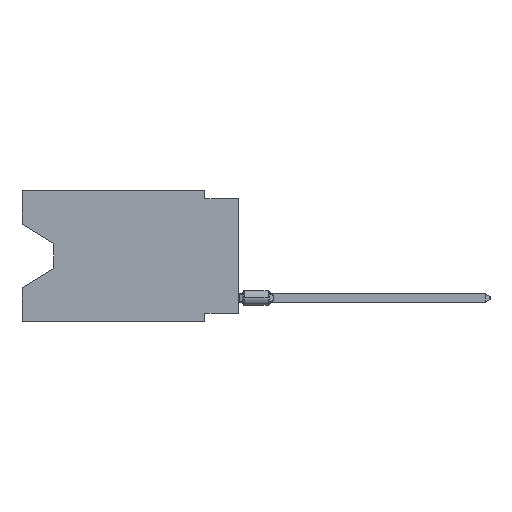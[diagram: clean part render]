
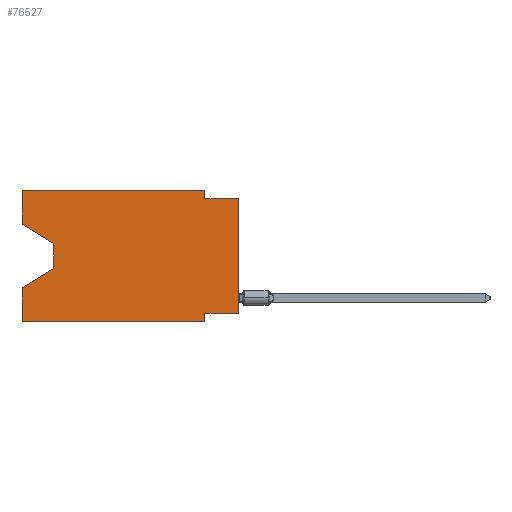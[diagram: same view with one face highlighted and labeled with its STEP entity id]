
A CAD part, left-side view. The second image highlights one B-rep face of the part: STEP entity #76527.
In plain terms, the highlighted planar face has unit normal (-1, 0, 0).
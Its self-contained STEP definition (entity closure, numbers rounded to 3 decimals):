
#252 = DIRECTION ( 'NONE',  ( 0., -1., 0. ) ) ;
#320 = DIRECTION ( 'NONE',  ( 0., 0., 1. ) ) ;
#883 = CARTESIAN_POINT ( 'NONE',  ( 0., 16.383, 0. ) ) ;
#2734 = VERTEX_POINT ( 'NONE', #69233 ) ;
#3400 = VERTEX_POINT ( 'NONE', #31147 ) ;
#4760 = CARTESIAN_POINT ( 'NONE',  ( 0., 13.97, -4.013 ) ) ;
#5034 = EDGE_CURVE ( 'NONE', #14132, #26590, #78920, .T. ) ;
#6052 = VECTOR ( 'NONE', #58578, 1000. ) ;
#8545 = EDGE_CURVE ( 'NONE', #2734, #3400, #18731, .T. ) ;
#8686 = EDGE_CURVE ( 'NONE', #66600, #31402, #77104, .T. ) ;
#9120 = FACE_OUTER_BOUND ( 'NONE', #32120, .T. ) ;
#9383 = CARTESIAN_POINT ( 'NONE',  ( 0., 16.383, -2.546 ) ) ;
#10279 = VERTEX_POINT ( 'NONE', #65061 ) ;
#11638 = ORIENTED_EDGE ( 'NONE', *, *, #46056, .F. ) ;
#11799 = CARTESIAN_POINT ( 'NONE',  ( 0., 16.383, -9.906 ) ) ;
#11933 = LINE ( 'NONE', #24694, #43469 ) ;
#11943 = CARTESIAN_POINT ( 'NONE',  ( 0., 2.54, -9.906 ) ) ;
#12550 = AXIS2_PLACEMENT_3D ( 'NONE', #46155, #47347, #40383 ) ;
#13216 = LINE ( 'NONE', #883, #72345 ) ;
#13653 = VERTEX_POINT ( 'NONE', #71259 ) ;
#14021 = DIRECTION ( 'NONE',  ( 0., 0., 1. ) ) ;
#14132 = VERTEX_POINT ( 'NONE', #9383 ) ;
#14523 = CARTESIAN_POINT ( 'NONE',  ( 0., 16.383, 0. ) ) ;
#14985 = CARTESIAN_POINT ( 'NONE',  ( 0., 16.383, -9.906 ) ) ;
#15037 = ORIENTED_EDGE ( 'NONE', *, *, #69292, .T. ) ;
#18731 = LINE ( 'NONE', #63143, #41501 ) ;
#20575 = EDGE_CURVE ( 'NONE', #66600, #42557, #48158, .T. ) ;
#20995 = ORIENTED_EDGE ( 'NONE', *, *, #8545, .F. ) ;
#21730 = ORIENTED_EDGE ( 'NONE', *, *, #49374, .T. ) ;
#22168 = ORIENTED_EDGE ( 'NONE', *, *, #8686, .T. ) ;
#23482 = DIRECTION ( 'NONE',  ( 0., 0., 1. ) ) ;
#23581 = EDGE_CURVE ( 'NONE', #80681, #2734, #27623, .T. ) ;
#23883 = CARTESIAN_POINT ( 'NONE',  ( 0., 2.54, 0. ) ) ;
#24074 = LINE ( 'NONE', #4760, #71920 ) ;
#24694 = CARTESIAN_POINT ( 'NONE',  ( 0., 13.97, -5.893 ) ) ;
#25001 = VECTOR ( 'NONE', #39782, 1000. ) ;
#25594 = VERTEX_POINT ( 'NONE', #27034 ) ;
#26219 = CARTESIAN_POINT ( 'NONE',  ( 0., 0., -9.271 ) ) ;
#26590 = VERTEX_POINT ( 'NONE', #40401 ) ;
#27034 = CARTESIAN_POINT ( 'NONE',  ( 0., 13.97, -5.893 ) ) ;
#27076 = VECTOR ( 'NONE', #62102, 1000. ) ;
#27623 = LINE ( 'NONE', #63812, #40417 ) ;
#28170 = ORIENTED_EDGE ( 'NONE', *, *, #51060, .T. ) ;
#28357 = CARTESIAN_POINT ( 'NONE',  ( 0., 16.383, -2.546 ) ) ;
#30069 = VECTOR ( 'NONE', #320, 1000. ) ;
#31147 = CARTESIAN_POINT ( 'NONE',  ( 0., 0., -0.635 ) ) ;
#31402 = VERTEX_POINT ( 'NONE', #54485 ) ;
#32120 = EDGE_LOOP ( 'NONE', ( #36645, #21730, #15037, #40315, #22168, #11638, #81163, #28170, #20995, #37287, #57094, #35617 ) ) ;
#35617 = ORIENTED_EDGE ( 'NONE', *, *, #55524, .F. ) ;
#36645 = ORIENTED_EDGE ( 'NONE', *, *, #5034, .T. ) ;
#37287 = ORIENTED_EDGE ( 'NONE', *, *, #23581, .F. ) ;
#37332 = LINE ( 'NONE', #68564, #30069 ) ;
#39782 = DIRECTION ( 'NONE',  ( 0., 1., 0. ) ) ;
#40315 = ORIENTED_EDGE ( 'NONE', *, *, #20575, .F. ) ;
#40383 = DIRECTION ( 'NONE',  ( 0., 0., -1. ) ) ;
#40401 = CARTESIAN_POINT ( 'NONE',  ( 0., 13.97, -4.013 ) ) ;
#40417 = VECTOR ( 'NONE', #58065, 1000. ) ;
#41501 = VECTOR ( 'NONE', #252, 1000. ) ;
#42437 = DIRECTION ( 'NONE',  ( 0., -1., 0. ) ) ;
#42557 = VERTEX_POINT ( 'NONE', #77464 ) ;
#43469 = VECTOR ( 'NONE', #74847, 1000. ) ;
#45945 = LINE ( 'NONE', #26219, #25001 ) ;
#46056 = EDGE_CURVE ( 'NONE', #64828, #31402, #68265, .T. ) ;
#46155 = CARTESIAN_POINT ( 'NONE',  ( 0., 16.383, 0. ) ) ;
#47347 = DIRECTION ( 'NONE',  ( 1., 0., 0. ) ) ;
#48158 = LINE ( 'NONE', #72816, #77491 ) ;
#49270 = VECTOR ( 'NONE', #42437, 1000. ) ;
#49374 = EDGE_CURVE ( 'NONE', #26590, #25594, #24074, .T. ) ;
#51060 = EDGE_CURVE ( 'NONE', #13653, #3400, #37332, .T. ) ;
#52389 = EDGE_CURVE ( 'NONE', #13653, #64828, #45945, .T. ) ;
#54485 = CARTESIAN_POINT ( 'NONE',  ( 0., 2.54, -9.906 ) ) ;
#55524 = EDGE_CURVE ( 'NONE', #14132, #10279, #13216, .T. ) ;
#57094 = ORIENTED_EDGE ( 'NONE', *, *, #60125, .F. ) ;
#58065 = DIRECTION ( 'NONE',  ( 0., 0., -1. ) ) ;
#58109 = LINE ( 'NONE', #14523, #49270 ) ;
#58578 = DIRECTION ( 'NONE',  ( 0., -1., 0. ) ) ;
#60125 = EDGE_CURVE ( 'NONE', #10279, #80681, #58109, .T. ) ;
#60577 = VECTOR ( 'NONE', #71529, 1000. ) ;
#62102 = DIRECTION ( 'NONE',  ( 0., 0., -1. ) ) ;
#63143 = CARTESIAN_POINT ( 'NONE',  ( 0., 0., -0.635 ) ) ;
#63548 = CARTESIAN_POINT ( 'NONE',  ( 0., 2.54, -9.271 ) ) ;
#63812 = CARTESIAN_POINT ( 'NONE',  ( 0., 2.54, 0. ) ) ;
#64828 = VERTEX_POINT ( 'NONE', #63548 ) ;
#65061 = CARTESIAN_POINT ( 'NONE',  ( 0., 16.383, 0. ) ) ;
#66600 = VERTEX_POINT ( 'NONE', #11799 ) ;
#68070 = DIRECTION ( 'NONE',  ( 0., 0., -1. ) ) ;
#68265 = LINE ( 'NONE', #11943, #27076 ) ;
#68564 = CARTESIAN_POINT ( 'NONE',  ( 0., 0., 0. ) ) ;
#69233 = CARTESIAN_POINT ( 'NONE',  ( 0., 2.54, -0.635 ) ) ;
#69292 = EDGE_CURVE ( 'NONE', #25594, #42557, #11933, .T. ) ;
#71259 = CARTESIAN_POINT ( 'NONE',  ( 0., 0., -9.271 ) ) ;
#71529 = DIRECTION ( 'NONE',  ( 0., -0.855, -0.519 ) ) ;
#71609 = PLANE ( 'NONE',  #12550 ) ;
#71920 = VECTOR ( 'NONE', #68070, 1000. ) ;
#72345 = VECTOR ( 'NONE', #14021, 1000. ) ;
#72816 = CARTESIAN_POINT ( 'NONE',  ( 0., 16.383, 0. ) ) ;
#74847 = DIRECTION ( 'NONE',  ( 0., 0.855, -0.519 ) ) ;
#76527 = ADVANCED_FACE ( 'NONE', ( #9120 ), #71609, .F. ) ;
#77104 = LINE ( 'NONE', #14985, #6052 ) ;
#77464 = CARTESIAN_POINT ( 'NONE',  ( 0., 16.383, -7.36 ) ) ;
#77491 = VECTOR ( 'NONE', #23482, 1000. ) ;
#78920 = LINE ( 'NONE', #28357, #60577 ) ;
#80681 = VERTEX_POINT ( 'NONE', #23883 ) ;
#81163 = ORIENTED_EDGE ( 'NONE', *, *, #52389, .F. ) ;
